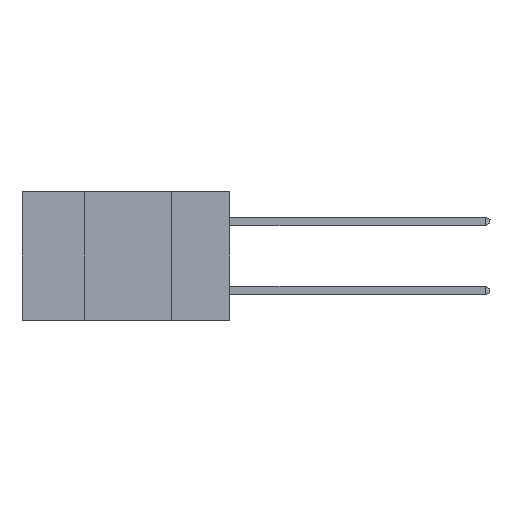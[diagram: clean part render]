
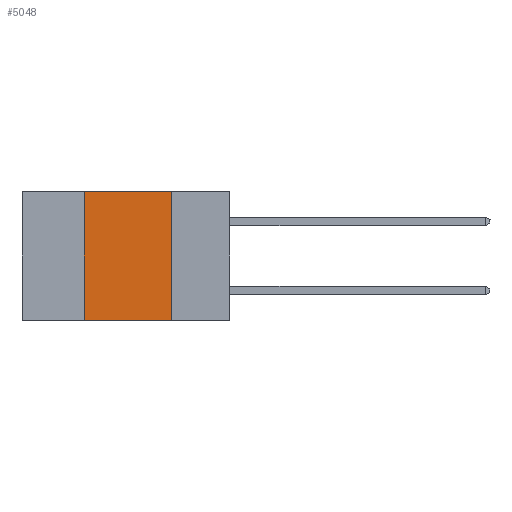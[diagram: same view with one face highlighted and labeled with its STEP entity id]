
A CAD part, left-side view. The second image highlights one B-rep face of the part: STEP entity #5048.
In plain terms, the highlighted planar face has unit normal (-1, 0, 0).
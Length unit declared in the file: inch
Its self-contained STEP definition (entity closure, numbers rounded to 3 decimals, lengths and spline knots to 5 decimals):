
#622 = PLANE ( 'NONE',  #4920 ) ;
#664 = CARTESIAN_POINT ( 'NONE',  ( 0., 0.42, -0.37 ) ) ;
#1764 = ORIENTED_EDGE ( 'NONE', *, *, #11617, .F. ) ;
#2131 = EDGE_LOOP ( 'NONE', ( #8390, #1764, #2659, #17605 ) ) ;
#2659 = ORIENTED_EDGE ( 'NONE', *, *, #8044, .F. ) ;
#3352 = VECTOR ( 'NONE', #6803, 39.37008 ) ;
#4219 = LINE ( 'NONE', #5848, #15382 ) ;
#4237 = VERTEX_POINT ( 'NONE', #15372 ) ;
#4920 = AXIS2_PLACEMENT_3D ( 'NONE', #14723, #6831, #11407 ) ;
#5048 = ADVANCED_FACE ( 'NONE', ( #13201 ), #622, .F. ) ;
#5848 = CARTESIAN_POINT ( 'NONE',  ( 0., 0.42, -0.37 ) ) ;
#6243 = CARTESIAN_POINT ( 'NONE',  ( 0., 0.42, 0. ) ) ;
#6357 = DIRECTION ( 'NONE',  ( 0., 0., -1. ) ) ;
#6479 = CARTESIAN_POINT ( 'NONE',  ( 0., 0.17, -0.37 ) ) ;
#6803 = DIRECTION ( 'NONE',  ( 0., -1., 0. ) ) ;
#6831 = DIRECTION ( 'NONE',  ( 1., 0., 0. ) ) ;
#8044 = EDGE_CURVE ( 'NONE', #15835, #11966, #4219, .T. ) ;
#8390 = ORIENTED_EDGE ( 'NONE', *, *, #13926, .F. ) ;
#9645 = LINE ( 'NONE', #19887, #16022 ) ;
#10144 = VERTEX_POINT ( 'NONE', #13897 ) ;
#10974 = LINE ( 'NONE', #19359, #3352 ) ;
#11394 = VECTOR ( 'NONE', #6357, 39.37008 ) ;
#11407 = DIRECTION ( 'NONE',  ( 0., 0., -1. ) ) ;
#11617 = EDGE_CURVE ( 'NONE', #11966, #10144, #10974, .T. ) ;
#11966 = VERTEX_POINT ( 'NONE', #6243 ) ;
#12227 = DIRECTION ( 'NONE',  ( 0., 0., 1. ) ) ;
#13201 = FACE_OUTER_BOUND ( 'NONE', #2131, .T. ) ;
#13697 = EDGE_CURVE ( 'NONE', #15835, #4237, #9645, .T. ) ;
#13897 = CARTESIAN_POINT ( 'NONE',  ( 0., 0.17, 0. ) ) ;
#13926 = EDGE_CURVE ( 'NONE', #10144, #4237, #14279, .T. ) ;
#14279 = LINE ( 'NONE', #6479, #11394 ) ;
#14723 = CARTESIAN_POINT ( 'NONE',  ( 0., 0.6, 0. ) ) ;
#15372 = CARTESIAN_POINT ( 'NONE',  ( 0., 0.17, -0.37 ) ) ;
#15382 = VECTOR ( 'NONE', #12227, 39.37008 ) ;
#15835 = VERTEX_POINT ( 'NONE', #664 ) ;
#16022 = VECTOR ( 'NONE', #19794, 39.37008 ) ;
#17605 = ORIENTED_EDGE ( 'NONE', *, *, #13697, .T. ) ;
#19359 = CARTESIAN_POINT ( 'NONE',  ( 0., 0.6, 0. ) ) ;
#19794 = DIRECTION ( 'NONE',  ( 0., -1., 0. ) ) ;
#19887 = CARTESIAN_POINT ( 'NONE',  ( 0., 0.6, -0.37 ) ) ;
